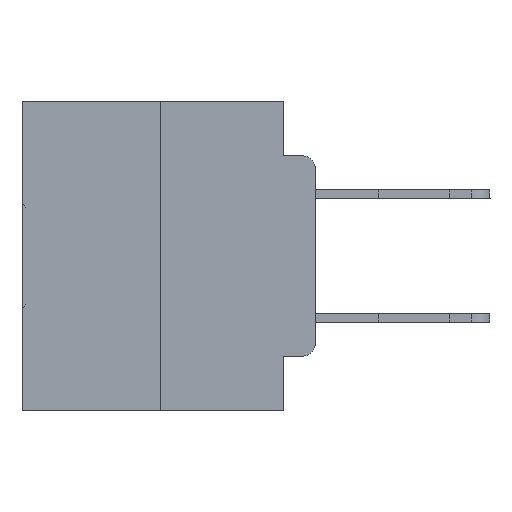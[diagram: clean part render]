
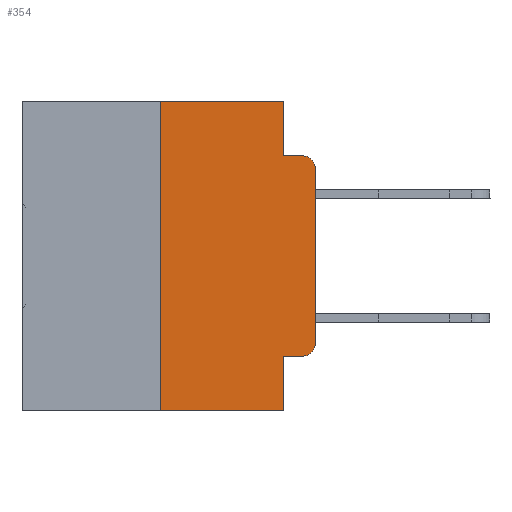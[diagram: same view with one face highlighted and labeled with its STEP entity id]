
A CAD part, left-side view. The second image highlights one B-rep face of the part: STEP entity #354.
In plain terms, the highlighted planar face has unit normal (-1, 0, 0).
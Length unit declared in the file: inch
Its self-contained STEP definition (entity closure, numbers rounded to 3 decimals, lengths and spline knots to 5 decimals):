
#354 = ADVANCED_FACE ( 'NONE', ( #22081 ), #18713, .F. ) ;
#1380 = CARTESIAN_POINT ( 'NONE',  ( 0., 0.02, -0.4115 ) ) ;
#1386 = VECTOR ( 'NONE', #22054, 39.37008 ) ;
#2126 = ORIENTED_EDGE ( 'NONE', *, *, #8696, .T. ) ;
#2234 = CARTESIAN_POINT ( 'NONE',  ( 0., 0.25, 0. ) ) ;
#2403 = AXIS2_PLACEMENT_3D ( 'NONE', #25638, #10557, #28172 ) ;
#2519 = CARTESIAN_POINT ( 'NONE',  ( 0., 0.051, -0.0885 ) ) ;
#2811 = ORIENTED_EDGE ( 'NONE', *, *, #28975, .T. ) ;
#5116 = CARTESIAN_POINT ( 'NONE',  ( 0., 0.25, 0. ) ) ;
#5316 = ORIENTED_EDGE ( 'NONE', *, *, #18898, .F. ) ;
#6802 = VECTOR ( 'NONE', #30707, 39.37008 ) ;
#7116 = VERTEX_POINT ( 'NONE', #17113 ) ;
#7141 = DIRECTION ( 'NONE',  ( 0., 0., -1. ) ) ;
#8499 = VECTOR ( 'NONE', #25373, 39.37008 ) ;
#8696 = EDGE_CURVE ( 'NONE', #25302, #15148, #16606, .T. ) ;
#9186 = VERTEX_POINT ( 'NONE', #2234 ) ;
#9287 = ORIENTED_EDGE ( 'NONE', *, *, #22818, .F. ) ;
#9570 = CARTESIAN_POINT ( 'NONE',  ( 0., 0.051, -0.4115 ) ) ;
#9880 = VERTEX_POINT ( 'NONE', #2519 ) ;
#10395 = CARTESIAN_POINT ( 'NONE',  ( 0., 0., -0.1085 ) ) ;
#10401 = EDGE_CURVE ( 'NONE', #16174, #25302, #13752, .T. ) ;
#10557 = DIRECTION ( 'NONE',  ( -1., 0., 0. ) ) ;
#10924 = CARTESIAN_POINT ( 'NONE',  ( 0., 0.051, 0. ) ) ;
#12149 = DIRECTION ( 'NONE',  ( 0., -1., 0. ) ) ;
#12242 = LINE ( 'NONE', #10924, #13025 ) ;
#12284 = DIRECTION ( 'NONE',  ( 0., -1., 0. ) ) ;
#13025 = VECTOR ( 'NONE', #13488, 39.37008 ) ;
#13191 = LINE ( 'NONE', #24819, #19111 ) ;
#13488 = DIRECTION ( 'NONE',  ( 0., 0., -1. ) ) ;
#13677 = ORIENTED_EDGE ( 'NONE', *, *, #27297, .F. ) ;
#13752 = LINE ( 'NONE', #9570, #27878 ) ;
#13846 = CARTESIAN_POINT ( 'NONE',  ( 0., 0.02, -0.1085 ) ) ;
#14397 = LINE ( 'NONE', #25692, #6802 ) ;
#14518 = VERTEX_POINT ( 'NONE', #10395 ) ;
#15148 = VERTEX_POINT ( 'NONE', #25350 ) ;
#16069 = LINE ( 'NONE', #5116, #8499 ) ;
#16174 = VERTEX_POINT ( 'NONE', #29893 ) ;
#16359 = DIRECTION ( 'NONE',  ( 0., 0., -1. ) ) ;
#16431 = VERTEX_POINT ( 'NONE', #30918 ) ;
#16568 = CARTESIAN_POINT ( 'NONE',  ( 0., 0.473, 0. ) ) ;
#16606 = CIRCLE ( 'NONE', #2403, 0.02 ) ;
#16885 = EDGE_LOOP ( 'NONE', ( #21506, #2811, #13677, #19217, #9287, #17247, #27069, #5316, #27872, #2126 ) ) ;
#16948 = DIRECTION ( 'NONE',  ( 1., 0., 0. ) ) ;
#16963 = VERTEX_POINT ( 'NONE', #30465 ) ;
#16979 = DIRECTION ( 'NONE',  ( 0., 0., -1. ) ) ;
#17113 = CARTESIAN_POINT ( 'NONE',  ( 0., 0.051, -0.5 ) ) ;
#17247 = ORIENTED_EDGE ( 'NONE', *, *, #20558, .F. ) ;
#17514 = LINE ( 'NONE', #29847, #29276 ) ;
#18713 = PLANE ( 'NONE',  #26390 ) ;
#18898 = EDGE_CURVE ( 'NONE', #16174, #7116, #12242, .T. ) ;
#18930 = CARTESIAN_POINT ( 'NONE',  ( 0., 0.25, -0.5 ) ) ;
#19111 = VECTOR ( 'NONE', #7141, 39.37008 ) ;
#19217 = ORIENTED_EDGE ( 'NONE', *, *, #22246, .F. ) ;
#19558 = CARTESIAN_POINT ( 'NONE',  ( 0., 0.051, -0.0885 ) ) ;
#20228 = VERTEX_POINT ( 'NONE', #18930 ) ;
#20558 = EDGE_CURVE ( 'NONE', #20228, #9186, #16069, .T. ) ;
#21506 = ORIENTED_EDGE ( 'NONE', *, *, #30622, .T. ) ;
#22054 = DIRECTION ( 'NONE',  ( 0., -1., 0. ) ) ;
#22081 = FACE_OUTER_BOUND ( 'NONE', #16885, .T. ) ;
#22215 = AXIS2_PLACEMENT_3D ( 'NONE', #13846, #31323, #16359 ) ;
#22246 = EDGE_CURVE ( 'NONE', #16431, #9880, #13191, .T. ) ;
#22818 = EDGE_CURVE ( 'NONE', #9186, #16431, #23381, .T. ) ;
#23381 = LINE ( 'NONE', #32381, #29258 ) ;
#23933 = CIRCLE ( 'NONE', #22215, 0.02 ) ;
#24819 = CARTESIAN_POINT ( 'NONE',  ( 0., 0.051, 0. ) ) ;
#25302 = VERTEX_POINT ( 'NONE', #1380 ) ;
#25350 = CARTESIAN_POINT ( 'NONE',  ( 0., 0., -0.3915 ) ) ;
#25373 = DIRECTION ( 'NONE',  ( 0., 0., 1. ) ) ;
#25416 = EDGE_CURVE ( 'NONE', #20228, #7116, #17514, .T. ) ;
#25638 = CARTESIAN_POINT ( 'NONE',  ( 0., 0.02, -0.3915 ) ) ;
#25692 = CARTESIAN_POINT ( 'NONE',  ( 0., 0., 0. ) ) ;
#26390 = AXIS2_PLACEMENT_3D ( 'NONE', #16568, #16948, #16979 ) ;
#27069 = ORIENTED_EDGE ( 'NONE', *, *, #25416, .T. ) ;
#27297 = EDGE_CURVE ( 'NONE', #9880, #16963, #27588, .T. ) ;
#27588 = LINE ( 'NONE', #19558, #1386 ) ;
#27872 = ORIENTED_EDGE ( 'NONE', *, *, #10401, .T. ) ;
#27878 = VECTOR ( 'NONE', #12149, 39.37008 ) ;
#28172 = DIRECTION ( 'NONE',  ( 0., 0., -1. ) ) ;
#28975 = EDGE_CURVE ( 'NONE', #14518, #16963, #23933, .T. ) ;
#29258 = VECTOR ( 'NONE', #29935, 39.37008 ) ;
#29276 = VECTOR ( 'NONE', #12284, 39.37008 ) ;
#29847 = CARTESIAN_POINT ( 'NONE',  ( 0., 0.473, -0.5 ) ) ;
#29893 = CARTESIAN_POINT ( 'NONE',  ( 0., 0.051, -0.4115 ) ) ;
#29935 = DIRECTION ( 'NONE',  ( 0., -1., 0. ) ) ;
#30465 = CARTESIAN_POINT ( 'NONE',  ( 0., 0.02, -0.0885 ) ) ;
#30622 = EDGE_CURVE ( 'NONE', #15148, #14518, #14397, .T. ) ;
#30707 = DIRECTION ( 'NONE',  ( 0., 0., 1. ) ) ;
#30918 = CARTESIAN_POINT ( 'NONE',  ( 0., 0.051, 0. ) ) ;
#31323 = DIRECTION ( 'NONE',  ( -1., 0., 0. ) ) ;
#32381 = CARTESIAN_POINT ( 'NONE',  ( 0., 0.473, 0. ) ) ;
